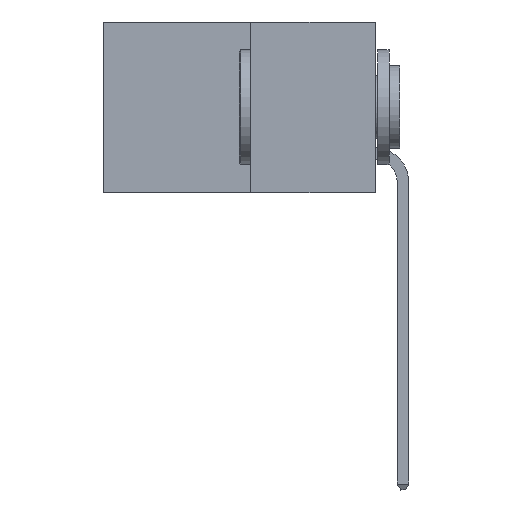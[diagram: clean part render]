
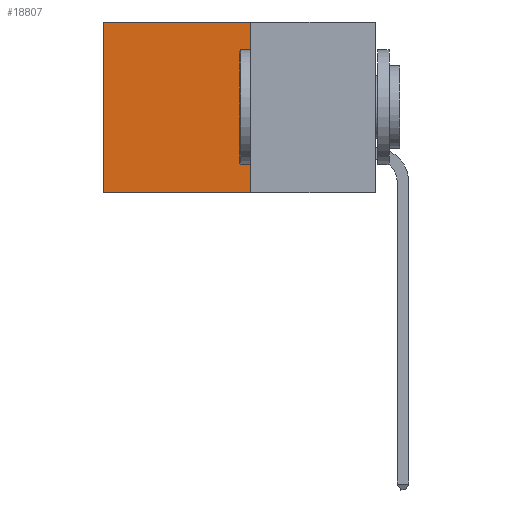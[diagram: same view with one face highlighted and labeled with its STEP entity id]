
A CAD part, left-side view. The second image highlights one B-rep face of the part: STEP entity #18807.
In plain terms, the highlighted planar face has unit normal (-1, 0, 0).
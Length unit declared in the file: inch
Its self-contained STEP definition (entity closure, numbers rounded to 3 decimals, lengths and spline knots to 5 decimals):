
#529 = EDGE_LOOP ( 'NONE', ( #1680, #7709, #17247, #5183 ) ) ;
#582 = VECTOR ( 'NONE', #8022, 39.37008 ) ;
#1680 = ORIENTED_EDGE ( 'NONE', *, *, #13009, .T. ) ;
#1805 = LINE ( 'NONE', #19208, #5582 ) ;
#1843 = DIRECTION ( 'NONE',  ( 0., 0., -1. ) ) ;
#2368 = CARTESIAN_POINT ( 'NONE',  ( 0.277, 0.27, -0.37 ) ) ;
#3162 = AXIS2_PLACEMENT_3D ( 'NONE', #12046, #17424, #6681 ) ;
#4229 = DIRECTION ( 'NONE',  ( 0., 0., -1. ) ) ;
#4872 = PLANE ( 'NONE',  #3162 ) ;
#5183 = ORIENTED_EDGE ( 'NONE', *, *, #16900, .T. ) ;
#5335 = VERTEX_POINT ( 'NONE', #10176 ) ;
#5496 = CARTESIAN_POINT ( 'NONE',  ( 0.277, 0.59, -0.37 ) ) ;
#5582 = VECTOR ( 'NONE', #10256, 39.37008 ) ;
#5931 = CARTESIAN_POINT ( 'NONE',  ( 0.277, 0.59, -0.37 ) ) ;
#6045 = VERTEX_POINT ( 'NONE', #22928 ) ;
#6207 = CARTESIAN_POINT ( 'NONE',  ( 0.277, 0.27, 0. ) ) ;
#6681 = DIRECTION ( 'NONE',  ( 0., 0., -1. ) ) ;
#7665 = VECTOR ( 'NONE', #4229, 39.37008 ) ;
#7709 = ORIENTED_EDGE ( 'NONE', *, *, #23088, .F. ) ;
#8022 = DIRECTION ( 'NONE',  ( 0., 1., 0. ) ) ;
#9062 = VERTEX_POINT ( 'NONE', #5931 ) ;
#10176 = CARTESIAN_POINT ( 'NONE',  ( 0.277, 0.59, 0. ) ) ;
#10256 = DIRECTION ( 'NONE',  ( 0., 1., 0. ) ) ;
#10285 = LINE ( 'NONE', #6207, #582 ) ;
#12046 = CARTESIAN_POINT ( 'NONE',  ( 0.277, 0.27, -0.37 ) ) ;
#13009 = EDGE_CURVE ( 'NONE', #5335, #9062, #22770, .T. ) ;
#14487 = VERTEX_POINT ( 'NONE', #17020 ) ;
#16900 = EDGE_CURVE ( 'NONE', #6045, #5335, #10285, .T. ) ;
#17020 = CARTESIAN_POINT ( 'NONE',  ( 0.277, 0.27, -0.37 ) ) ;
#17247 = ORIENTED_EDGE ( 'NONE', *, *, #18552, .F. ) ;
#17424 = DIRECTION ( 'NONE',  ( 1., 0., 0. ) ) ;
#18552 = EDGE_CURVE ( 'NONE', #6045, #14487, #21990, .T. ) ;
#18807 = ADVANCED_FACE ( 'NONE', ( #20381 ), #4872, .F. ) ;
#19208 = CARTESIAN_POINT ( 'NONE',  ( 0.277, 0.27, -0.37 ) ) ;
#20381 = FACE_OUTER_BOUND ( 'NONE', #529, .T. ) ;
#21990 = LINE ( 'NONE', #2368, #7665 ) ;
#22229 = VECTOR ( 'NONE', #1843, 39.37008 ) ;
#22770 = LINE ( 'NONE', #5496, #22229 ) ;
#22928 = CARTESIAN_POINT ( 'NONE',  ( 0.277, 0.27, 0. ) ) ;
#23088 = EDGE_CURVE ( 'NONE', #14487, #9062, #1805, .T. ) ;
